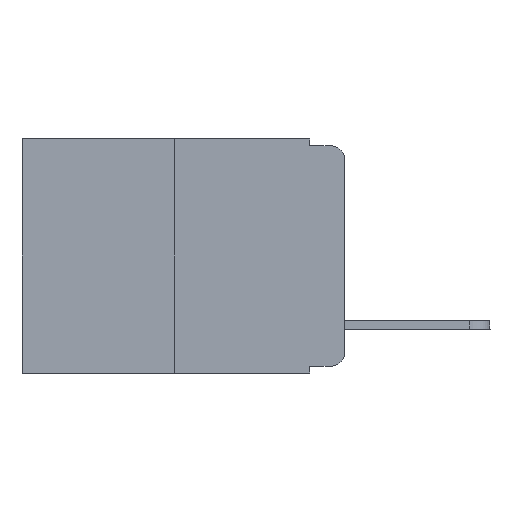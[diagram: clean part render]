
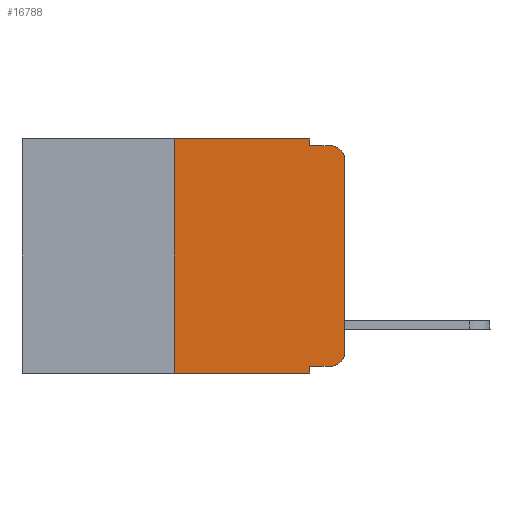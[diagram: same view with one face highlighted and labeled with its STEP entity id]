
A CAD part, left-side view. The second image highlights one B-rep face of the part: STEP entity #16788.
In plain terms, the highlighted planar face has unit normal (-1, 0, 0).
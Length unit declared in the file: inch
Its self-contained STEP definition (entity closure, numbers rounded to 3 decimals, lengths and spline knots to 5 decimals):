
#271 = CIRCLE ( 'NONE', #683, 0.02 ) ;
#376 = DIRECTION ( 'NONE',  ( 0., -1., 0. ) ) ;
#485 = VECTOR ( 'NONE', #9319, 39.37008 ) ;
#683 = AXIS2_PLACEMENT_3D ( 'NONE', #1465, #23462, #2194 ) ;
#802 = ORIENTED_EDGE ( 'NONE', *, *, #19617, .F. ) ;
#1075 = ORIENTED_EDGE ( 'NONE', *, *, #5841, .F. ) ;
#1374 = ORIENTED_EDGE ( 'NONE', *, *, #22114, .T. ) ;
#1465 = CARTESIAN_POINT ( 'NONE',  ( 0., 0.02, -0.313 ) ) ;
#1783 = CARTESIAN_POINT ( 'NONE',  ( 0., 0.25, -0.343 ) ) ;
#1854 = LINE ( 'NONE', #11749, #7357 ) ;
#2194 = DIRECTION ( 'NONE',  ( 0., 0., -1. ) ) ;
#3192 = LINE ( 'NONE', #9155, #6336 ) ;
#3241 = ORIENTED_EDGE ( 'NONE', *, *, #19259, .F. ) ;
#3286 = LINE ( 'NONE', #16830, #19150 ) ;
#3437 = VERTEX_POINT ( 'NONE', #19001 ) ;
#3471 = LINE ( 'NONE', #18915, #485 ) ;
#3492 = VERTEX_POINT ( 'NONE', #1783 ) ;
#3562 = CARTESIAN_POINT ( 'NONE',  ( 0., 0.25, 0. ) ) ;
#3872 = LINE ( 'NONE', #24778, #22731 ) ;
#4189 = CARTESIAN_POINT ( 'NONE',  ( 0., 0.473, 0. ) ) ;
#4713 = VERTEX_POINT ( 'NONE', #24711 ) ;
#4722 = VERTEX_POINT ( 'NONE', #3562 ) ;
#5247 = EDGE_CURVE ( 'NONE', #3437, #16866, #13424, .T. ) ;
#5469 = CARTESIAN_POINT ( 'NONE',  ( 0., 0.473, 0. ) ) ;
#5722 = CARTESIAN_POINT ( 'NONE',  ( 0., 0.051, -0.01 ) ) ;
#5841 = EDGE_CURVE ( 'NONE', #22577, #6577, #1854, .T. ) ;
#6271 = EDGE_CURVE ( 'NONE', #3492, #4722, #3471, .T. ) ;
#6336 = VECTOR ( 'NONE', #24591, 39.37008 ) ;
#6364 = VERTEX_POINT ( 'NONE', #6842 ) ;
#6577 = VERTEX_POINT ( 'NONE', #15192 ) ;
#6842 = CARTESIAN_POINT ( 'NONE',  ( 0., 0.051, -0.333 ) ) ;
#7357 = VECTOR ( 'NONE', #9594, 39.37008 ) ;
#8026 = EDGE_CURVE ( 'NONE', #3492, #4713, #10289, .T. ) ;
#8394 = DIRECTION ( 'NONE',  ( 0., -1., 0. ) ) ;
#8567 = EDGE_LOOP ( 'NONE', ( #1374, #12054, #3241, #1075, #9768, #22980, #21487, #802, #10008, #14641 ) ) ;
#9000 = DIRECTION ( 'NONE',  ( -1., 0., 0. ) ) ;
#9155 = CARTESIAN_POINT ( 'NONE',  ( 0., 0., 0. ) ) ;
#9158 = LINE ( 'NONE', #5722, #13917 ) ;
#9319 = DIRECTION ( 'NONE',  ( 0., 0., 1. ) ) ;
#9520 = FACE_OUTER_BOUND ( 'NONE', #8567, .T. ) ;
#9594 = DIRECTION ( 'NONE',  ( 0., 0., -1. ) ) ;
#9768 = ORIENTED_EDGE ( 'NONE', *, *, #23671, .F. ) ;
#9769 = AXIS2_PLACEMENT_3D ( 'NONE', #15185, #9000, #24307 ) ;
#10008 = ORIENTED_EDGE ( 'NONE', *, *, #18284, .T. ) ;
#10289 = LINE ( 'NONE', #17870, #18844 ) ;
#11749 = CARTESIAN_POINT ( 'NONE',  ( 0., 0.051, 0. ) ) ;
#12054 = ORIENTED_EDGE ( 'NONE', *, *, #5247, .T. ) ;
#12943 = DIRECTION ( 'NONE',  ( 0., 0., -1. ) ) ;
#13080 = VERTEX_POINT ( 'NONE', #16546 ) ;
#13424 = CIRCLE ( 'NONE', #9769, 0.02 ) ;
#13917 = VECTOR ( 'NONE', #24593, 39.37008 ) ;
#14641 = ORIENTED_EDGE ( 'NONE', *, *, #22995, .T. ) ;
#15185 = CARTESIAN_POINT ( 'NONE',  ( 0., 0.02, -0.03 ) ) ;
#15192 = CARTESIAN_POINT ( 'NONE',  ( 0., 0.051, -0.01 ) ) ;
#16546 = CARTESIAN_POINT ( 'NONE',  ( 0., 0., -0.313 ) ) ;
#16788 = ADVANCED_FACE ( 'NONE', ( #9520 ), #22794, .F. ) ;
#16830 = CARTESIAN_POINT ( 'NONE',  ( 0., 0.051, 0. ) ) ;
#16866 = VERTEX_POINT ( 'NONE', #21879 ) ;
#16960 = CARTESIAN_POINT ( 'NONE',  ( 0., 0.051, 0. ) ) ;
#17239 = DIRECTION ( 'NONE',  ( 1., 0., 0. ) ) ;
#17427 = DIRECTION ( 'NONE',  ( 0., -1., 0. ) ) ;
#17732 = VERTEX_POINT ( 'NONE', #18850 ) ;
#17870 = CARTESIAN_POINT ( 'NONE',  ( 0., 0.473, -0.343 ) ) ;
#18284 = EDGE_CURVE ( 'NONE', #6364, #17732, #3872, .T. ) ;
#18681 = AXIS2_PLACEMENT_3D ( 'NONE', #5469, #17239, #21147 ) ;
#18844 = VECTOR ( 'NONE', #8394, 39.37008 ) ;
#18850 = CARTESIAN_POINT ( 'NONE',  ( 0., 0.02, -0.333 ) ) ;
#18915 = CARTESIAN_POINT ( 'NONE',  ( 0., 0.25, 0. ) ) ;
#19001 = CARTESIAN_POINT ( 'NONE',  ( 0., 0., -0.03 ) ) ;
#19150 = VECTOR ( 'NONE', #12943, 39.37008 ) ;
#19259 = EDGE_CURVE ( 'NONE', #6577, #16866, #9158, .T. ) ;
#19617 = EDGE_CURVE ( 'NONE', #6364, #4713, #3286, .T. ) ;
#21147 = DIRECTION ( 'NONE',  ( 0., 0., -1. ) ) ;
#21487 = ORIENTED_EDGE ( 'NONE', *, *, #8026, .T. ) ;
#21879 = CARTESIAN_POINT ( 'NONE',  ( 0., 0.02, -0.01 ) ) ;
#22114 = EDGE_CURVE ( 'NONE', #13080, #3437, #3192, .T. ) ;
#22577 = VERTEX_POINT ( 'NONE', #16960 ) ;
#22731 = VECTOR ( 'NONE', #17427, 39.37008 ) ;
#22794 = PLANE ( 'NONE',  #18681 ) ;
#22980 = ORIENTED_EDGE ( 'NONE', *, *, #6271, .F. ) ;
#22995 = EDGE_CURVE ( 'NONE', #17732, #13080, #271, .T. ) ;
#23328 = VECTOR ( 'NONE', #376, 39.37008 ) ;
#23462 = DIRECTION ( 'NONE',  ( -1., 0., 0. ) ) ;
#23671 = EDGE_CURVE ( 'NONE', #4722, #22577, #24062, .T. ) ;
#24062 = LINE ( 'NONE', #4189, #23328 ) ;
#24307 = DIRECTION ( 'NONE',  ( 0., 0., -1. ) ) ;
#24591 = DIRECTION ( 'NONE',  ( 0., 0., 1. ) ) ;
#24593 = DIRECTION ( 'NONE',  ( 0., -1., 0. ) ) ;
#24711 = CARTESIAN_POINT ( 'NONE',  ( 0., 0.051, -0.343 ) ) ;
#24778 = CARTESIAN_POINT ( 'NONE',  ( 0., 0.051, -0.333 ) ) ;
